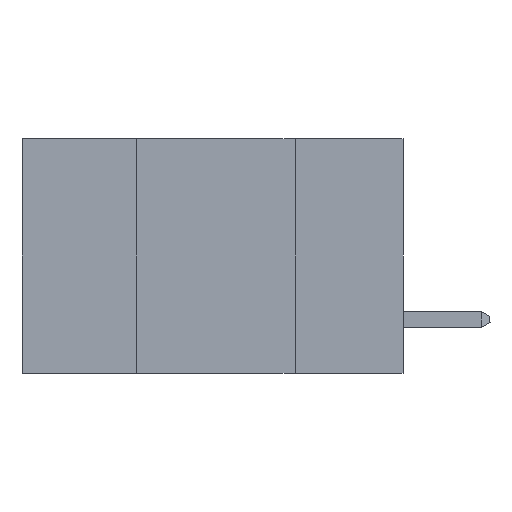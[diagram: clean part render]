
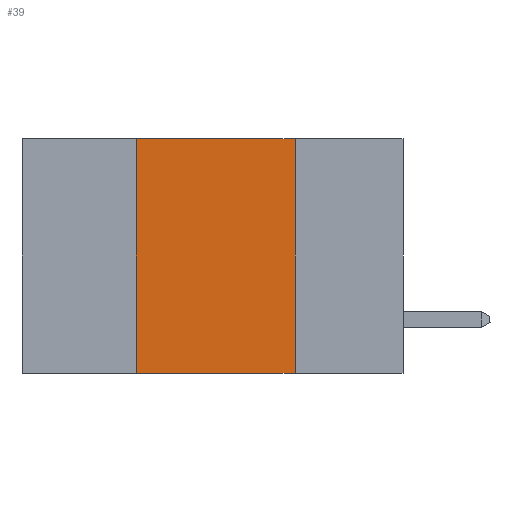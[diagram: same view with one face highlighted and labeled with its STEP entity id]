
A CAD part, left-side view. The second image highlights one B-rep face of the part: STEP entity #39.
In plain terms, the highlighted planar face has unit normal (-1, 0, 0).
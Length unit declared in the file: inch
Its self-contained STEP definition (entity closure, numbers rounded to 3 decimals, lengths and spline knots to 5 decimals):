
#39 = ADVANCED_FACE ( 'NONE', ( #12708 ), #1480, .F. ) ;
#126 = DIRECTION ( 'NONE',  ( 0., 0., -1. ) ) ;
#353 = EDGE_LOOP ( 'NONE', ( #11627, #16630, #8471, #790 ) ) ;
#790 = ORIENTED_EDGE ( 'NONE', *, *, #6975, .T. ) ;
#1480 = PLANE ( 'NONE',  #4073 ) ;
#1613 = CARTESIAN_POINT ( 'NONE',  ( 0., 0.17, 0. ) ) ;
#2135 = LINE ( 'NONE', #8229, #10318 ) ;
#2779 = DIRECTION ( 'NONE',  ( 0., -1., 0. ) ) ;
#3312 = CARTESIAN_POINT ( 'NONE',  ( 0., 0.42, -0.37 ) ) ;
#3519 = DIRECTION ( 'NONE',  ( 0., 0., 1. ) ) ;
#4073 = AXIS2_PLACEMENT_3D ( 'NONE', #11798, #6635, #126 ) ;
#4216 = DIRECTION ( 'NONE',  ( 0., 0., -1. ) ) ;
#4702 = VERTEX_POINT ( 'NONE', #9150 ) ;
#5200 = LINE ( 'NONE', #6078, #8053 ) ;
#6078 = CARTESIAN_POINT ( 'NONE',  ( 0., 0.42, 0. ) ) ;
#6079 = VECTOR ( 'NONE', #15534, 39.37008 ) ;
#6635 = DIRECTION ( 'NONE',  ( 1., 0., 0. ) ) ;
#6901 = LINE ( 'NONE', #10338, #6079 ) ;
#6975 = EDGE_CURVE ( 'NONE', #8073, #4702, #11763, .T. ) ;
#8041 = EDGE_CURVE ( 'NONE', #9374, #4702, #2135, .T. ) ;
#8053 = VECTOR ( 'NONE', #3519, 39.37008 ) ;
#8073 = VERTEX_POINT ( 'NONE', #3312 ) ;
#8229 = CARTESIAN_POINT ( 'NONE',  ( 0., 0.17, 0. ) ) ;
#8471 = ORIENTED_EDGE ( 'NONE', *, *, #13127, .F. ) ;
#9150 = CARTESIAN_POINT ( 'NONE',  ( 0., 0.17, -0.37 ) ) ;
#9374 = VERTEX_POINT ( 'NONE', #1613 ) ;
#10318 = VECTOR ( 'NONE', #4216, 39.37008 ) ;
#10338 = CARTESIAN_POINT ( 'NONE',  ( 0., 0.6, 0. ) ) ;
#11276 = CARTESIAN_POINT ( 'NONE',  ( 0., 0.42, 0. ) ) ;
#11627 = ORIENTED_EDGE ( 'NONE', *, *, #8041, .F. ) ;
#11675 = EDGE_CURVE ( 'NONE', #14505, #9374, #6901, .T. ) ;
#11694 = CARTESIAN_POINT ( 'NONE',  ( 0., 0.6, -0.37 ) ) ;
#11763 = LINE ( 'NONE', #11694, #14386 ) ;
#11798 = CARTESIAN_POINT ( 'NONE',  ( 0., 0.6, 0. ) ) ;
#12708 = FACE_OUTER_BOUND ( 'NONE', #353, .T. ) ;
#13127 = EDGE_CURVE ( 'NONE', #8073, #14505, #5200, .T. ) ;
#14386 = VECTOR ( 'NONE', #2779, 39.37008 ) ;
#14505 = VERTEX_POINT ( 'NONE', #11276 ) ;
#15534 = DIRECTION ( 'NONE',  ( 0., -1., 0. ) ) ;
#16630 = ORIENTED_EDGE ( 'NONE', *, *, #11675, .F. ) ;
